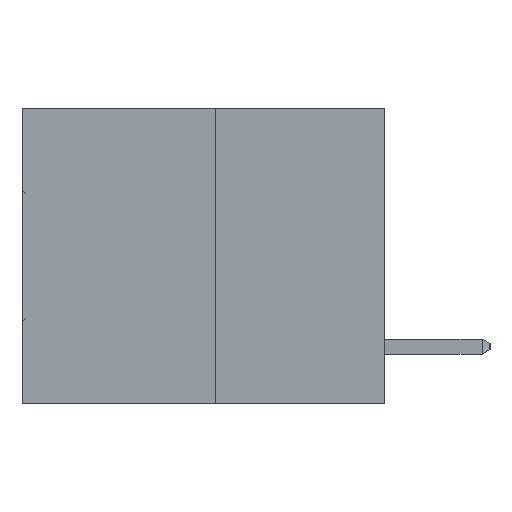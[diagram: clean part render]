
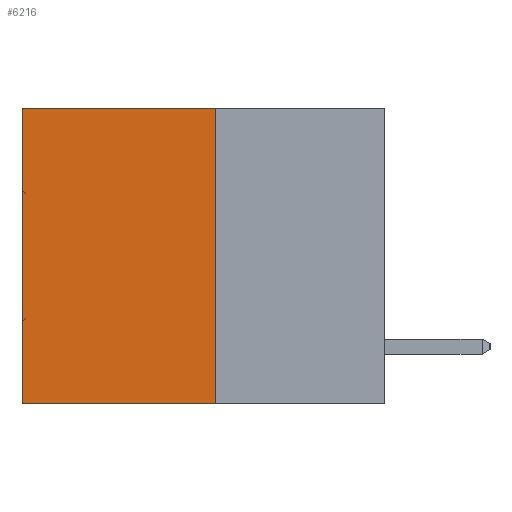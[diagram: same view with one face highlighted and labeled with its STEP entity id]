
A CAD part, left-side view. The second image highlights one B-rep face of the part: STEP entity #6216.
In plain terms, the highlighted planar face has unit normal (-1, 0, 0).
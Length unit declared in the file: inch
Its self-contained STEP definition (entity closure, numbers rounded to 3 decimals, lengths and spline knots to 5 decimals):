
#194 = PLANE ( 'NONE',  #18210 ) ;
#501 = ORIENTED_EDGE ( 'NONE', *, *, #31835, .T. ) ;
#946 = CARTESIAN_POINT ( 'NONE',  ( 0.3165, 0.28, -0.49 ) ) ;
#1629 = CARTESIAN_POINT ( 'NONE',  ( 0.3165, 0.6, -0.49 ) ) ;
#1700 = DIRECTION ( 'NONE',  ( 0., 1., 0. ) ) ;
#4269 = EDGE_CURVE ( 'NONE', #21445, #12020, #20336, .T. ) ;
#4981 = CARTESIAN_POINT ( 'NONE',  ( 0.3165, 0.28, -0.49 ) ) ;
#5235 = CARTESIAN_POINT ( 'NONE',  ( 0.3165, 0.28, -0.49 ) ) ;
#5674 = DIRECTION ( 'NONE',  ( 0., 0., -1. ) ) ;
#6053 = FACE_OUTER_BOUND ( 'NONE', #25101, .T. ) ;
#6216 = ADVANCED_FACE ( 'NONE', ( #6053 ), #194, .F. ) ;
#7787 = CARTESIAN_POINT ( 'NONE',  ( 0.3165, 0.28, 0. ) ) ;
#8100 = DIRECTION ( 'NONE',  ( 0., 0., -1. ) ) ;
#9022 = CARTESIAN_POINT ( 'NONE',  ( 0.3165, 0.28, -0.49 ) ) ;
#11680 = VERTEX_POINT ( 'NONE', #4981 ) ;
#12020 = VERTEX_POINT ( 'NONE', #33152 ) ;
#15767 = CARTESIAN_POINT ( 'NONE',  ( 0.3165, 0.6, -0.49 ) ) ;
#16478 = LINE ( 'NONE', #15767, #30261 ) ;
#18210 = AXIS2_PLACEMENT_3D ( 'NONE', #5235, #23293, #5674 ) ;
#18233 = LINE ( 'NONE', #9022, #30387 ) ;
#20300 = CARTESIAN_POINT ( 'NONE',  ( 0.3165, 0.28, 0. ) ) ;
#20336 = LINE ( 'NONE', #7787, #26824 ) ;
#20727 = VERTEX_POINT ( 'NONE', #1629 ) ;
#20728 = ORIENTED_EDGE ( 'NONE', *, *, #4269, .T. ) ;
#21445 = VERTEX_POINT ( 'NONE', #20300 ) ;
#23293 = DIRECTION ( 'NONE',  ( 1., 0., 0. ) ) ;
#25101 = EDGE_LOOP ( 'NONE', ( #501, #31440, #27420, #20728 ) ) ;
#25972 = DIRECTION ( 'NONE',  ( 0., 1., 0. ) ) ;
#26549 = DIRECTION ( 'NONE',  ( 0., 0., -1. ) ) ;
#26824 = VECTOR ( 'NONE', #25972, 39.37008 ) ;
#27101 = EDGE_CURVE ( 'NONE', #21445, #11680, #32560, .T. ) ;
#27420 = ORIENTED_EDGE ( 'NONE', *, *, #27101, .F. ) ;
#29781 = VECTOR ( 'NONE', #26549, 39.37008 ) ;
#30261 = VECTOR ( 'NONE', #8100, 39.37008 ) ;
#30387 = VECTOR ( 'NONE', #1700, 39.37008 ) ;
#30482 = EDGE_CURVE ( 'NONE', #11680, #20727, #18233, .T. ) ;
#31440 = ORIENTED_EDGE ( 'NONE', *, *, #30482, .F. ) ;
#31835 = EDGE_CURVE ( 'NONE', #12020, #20727, #16478, .T. ) ;
#32560 = LINE ( 'NONE', #946, #29781 ) ;
#33152 = CARTESIAN_POINT ( 'NONE',  ( 0.3165, 0.6, 0. ) ) ;
